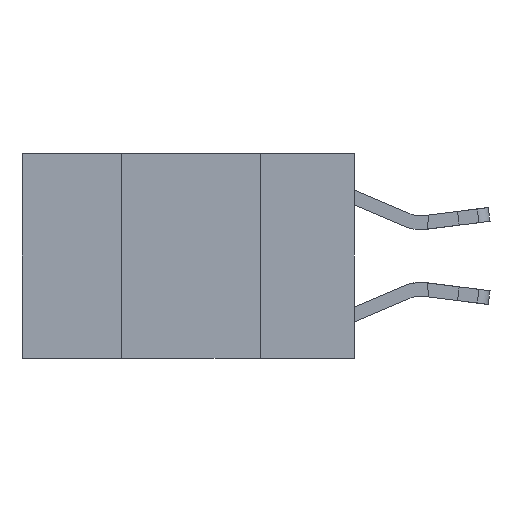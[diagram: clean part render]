
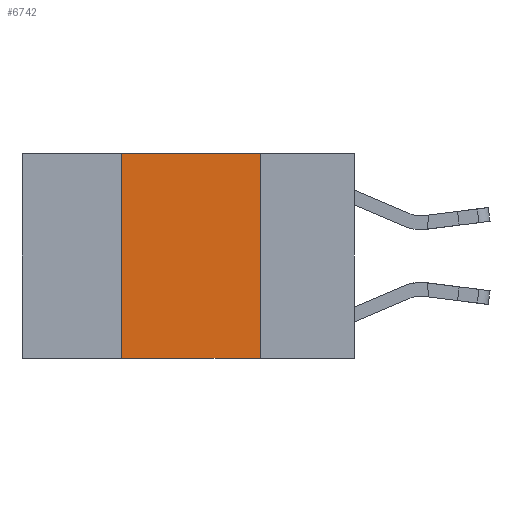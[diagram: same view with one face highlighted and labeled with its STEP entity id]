
A CAD part, left-side view. The second image highlights one B-rep face of the part: STEP entity #6742.
In plain terms, the highlighted planar face has unit normal (-1, 0, 0).
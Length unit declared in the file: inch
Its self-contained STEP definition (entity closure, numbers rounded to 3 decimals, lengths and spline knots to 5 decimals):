
#852 = AXIS2_PLACEMENT_3D ( 'NONE', #1742, #5903, #24912 ) ;
#1742 = CARTESIAN_POINT ( 'NONE',  ( 0., 0.6, 0. ) ) ;
#1921 = LINE ( 'NONE', #6344, #3190 ) ;
#2334 = VERTEX_POINT ( 'NONE', #9318 ) ;
#3190 = VECTOR ( 'NONE', #17833, 39.37008 ) ;
#3434 = VERTEX_POINT ( 'NONE', #23473 ) ;
#5047 = LINE ( 'NONE', #15347, #17309 ) ;
#5903 = DIRECTION ( 'NONE',  ( 1., 0., 0. ) ) ;
#6344 = CARTESIAN_POINT ( 'NONE',  ( 0., 0.17, 0. ) ) ;
#6502 = CARTESIAN_POINT ( 'NONE',  ( 0., 0.42, 0. ) ) ;
#6742 = ADVANCED_FACE ( 'NONE', ( #21811 ), #23639, .F. ) ;
#7476 = LINE ( 'NONE', #19490, #23188 ) ;
#9318 = CARTESIAN_POINT ( 'NONE',  ( 0., 0.17, 0. ) ) ;
#10687 = EDGE_CURVE ( 'NONE', #15742, #2334, #5047, .T. ) ;
#10717 = ORIENTED_EDGE ( 'NONE', *, *, #21806, .T. ) ;
#11363 = CARTESIAN_POINT ( 'NONE',  ( 0., 0.42, -0.37 ) ) ;
#11614 = EDGE_CURVE ( 'NONE', #2334, #3434, #1921, .T. ) ;
#12276 = VERTEX_POINT ( 'NONE', #11363 ) ;
#12599 = CARTESIAN_POINT ( 'NONE',  ( 0., 0.42, 0. ) ) ;
#13925 = LINE ( 'NONE', #6502, #22176 ) ;
#14682 = ORIENTED_EDGE ( 'NONE', *, *, #10687, .F. ) ;
#14916 = DIRECTION ( 'NONE',  ( 0., -1., 0. ) ) ;
#15347 = CARTESIAN_POINT ( 'NONE',  ( 0., 0.6, 0. ) ) ;
#15742 = VERTEX_POINT ( 'NONE', #12599 ) ;
#17050 = DIRECTION ( 'NONE',  ( 0., -1., 0. ) ) ;
#17081 = EDGE_CURVE ( 'NONE', #12276, #15742, #13925, .T. ) ;
#17309 = VECTOR ( 'NONE', #17050, 39.37008 ) ;
#17833 = DIRECTION ( 'NONE',  ( 0., 0., -1. ) ) ;
#19490 = CARTESIAN_POINT ( 'NONE',  ( 0., 0.6, -0.37 ) ) ;
#21368 = ORIENTED_EDGE ( 'NONE', *, *, #17081, .F. ) ;
#21806 = EDGE_CURVE ( 'NONE', #12276, #3434, #7476, .T. ) ;
#21811 = FACE_OUTER_BOUND ( 'NONE', #25254, .T. ) ;
#22176 = VECTOR ( 'NONE', #22397, 39.37008 ) ;
#22397 = DIRECTION ( 'NONE',  ( 0., 0., 1. ) ) ;
#23188 = VECTOR ( 'NONE', #14916, 39.37008 ) ;
#23473 = CARTESIAN_POINT ( 'NONE',  ( 0., 0.17, -0.37 ) ) ;
#23639 = PLANE ( 'NONE',  #852 ) ;
#23711 = ORIENTED_EDGE ( 'NONE', *, *, #11614, .F. ) ;
#24912 = DIRECTION ( 'NONE',  ( 0., 0., -1. ) ) ;
#25254 = EDGE_LOOP ( 'NONE', ( #23711, #14682, #21368, #10717 ) ) ;
